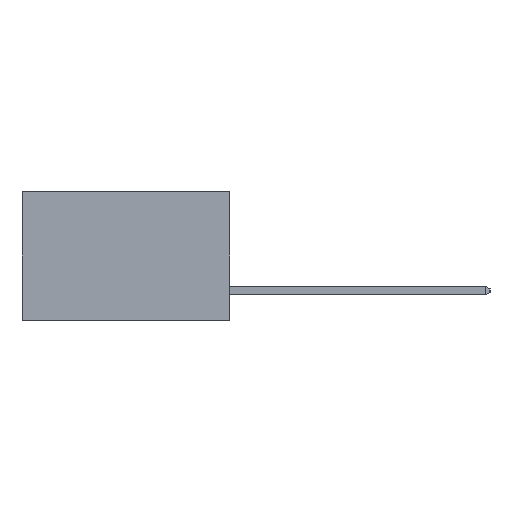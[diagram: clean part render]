
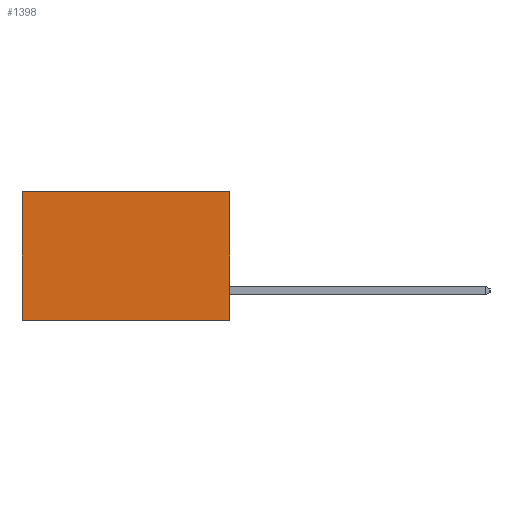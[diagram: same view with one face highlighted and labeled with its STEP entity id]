
A CAD part, left-side view. The second image highlights one B-rep face of the part: STEP entity #1398.
In plain terms, the highlighted planar face has unit normal (-1, 0, 0).
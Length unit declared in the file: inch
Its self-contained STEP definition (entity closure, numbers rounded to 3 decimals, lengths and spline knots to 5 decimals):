
#417 = VECTOR ( 'NONE', #8253, 39.37008 ) ;
#487 = VERTEX_POINT ( 'NONE', #13891 ) ;
#852 = DIRECTION ( 'NONE',  ( 1., 0., 0. ) ) ;
#1398 = ADVANCED_FACE ( 'NONE', ( #6177 ), #13067, .F. ) ;
#2535 = EDGE_CURVE ( 'NONE', #8835, #487, #9398, .T. ) ;
#2739 = CARTESIAN_POINT ( 'NONE',  ( 0.298, 0.6, 0. ) ) ;
#2903 = CARTESIAN_POINT ( 'NONE',  ( 0.298, 0., 0. ) ) ;
#3186 = DIRECTION ( 'NONE',  ( 0., 1., 0. ) ) ;
#3424 = CARTESIAN_POINT ( 'NONE',  ( 0.298, 0., -0.37 ) ) ;
#4758 = VECTOR ( 'NONE', #21956, 39.37008 ) ;
#6177 = FACE_OUTER_BOUND ( 'NONE', #17971, .T. ) ;
#6986 = DIRECTION ( 'NONE',  ( 0., 1., 0. ) ) ;
#8253 = DIRECTION ( 'NONE',  ( 0., 0., -1. ) ) ;
#8378 = LINE ( 'NONE', #17094, #21427 ) ;
#8835 = VERTEX_POINT ( 'NONE', #2739 ) ;
#9398 = LINE ( 'NONE', #10047, #4758 ) ;
#10047 = CARTESIAN_POINT ( 'NONE',  ( 0.298, 0.6, 0. ) ) ;
#11746 = EDGE_CURVE ( 'NONE', #14598, #8835, #8378, .T. ) ;
#12143 = ORIENTED_EDGE ( 'NONE', *, *, #2535, .T. ) ;
#13067 = PLANE ( 'NONE',  #20185 ) ;
#13843 = LINE ( 'NONE', #2903, #417 ) ;
#13891 = CARTESIAN_POINT ( 'NONE',  ( 0.298, 0.6, -0.37 ) ) ;
#13917 = VERTEX_POINT ( 'NONE', #20762 ) ;
#14598 = VERTEX_POINT ( 'NONE', #19367 ) ;
#14672 = ORIENTED_EDGE ( 'NONE', *, *, #11746, .T. ) ;
#16327 = EDGE_CURVE ( 'NONE', #13917, #487, #21034, .T. ) ;
#17094 = CARTESIAN_POINT ( 'NONE',  ( 0.298, 0., 0. ) ) ;
#17129 = DIRECTION ( 'NONE',  ( 0., 0., -1. ) ) ;
#17558 = ORIENTED_EDGE ( 'NONE', *, *, #16327, .F. ) ;
#17971 = EDGE_LOOP ( 'NONE', ( #12143, #17558, #21007, #14672 ) ) ;
#18164 = EDGE_CURVE ( 'NONE', #14598, #13917, #13843, .T. ) ;
#19367 = CARTESIAN_POINT ( 'NONE',  ( 0.298, 0., 0. ) ) ;
#20185 = AXIS2_PLACEMENT_3D ( 'NONE', #21939, #852, #17129 ) ;
#20543 = VECTOR ( 'NONE', #6986, 39.37008 ) ;
#20762 = CARTESIAN_POINT ( 'NONE',  ( 0.298, 0., -0.37 ) ) ;
#21007 = ORIENTED_EDGE ( 'NONE', *, *, #18164, .F. ) ;
#21034 = LINE ( 'NONE', #3424, #20543 ) ;
#21427 = VECTOR ( 'NONE', #3186, 39.37008 ) ;
#21939 = CARTESIAN_POINT ( 'NONE',  ( 0.298, 0., 0. ) ) ;
#21956 = DIRECTION ( 'NONE',  ( 0., 0., -1. ) ) ;
